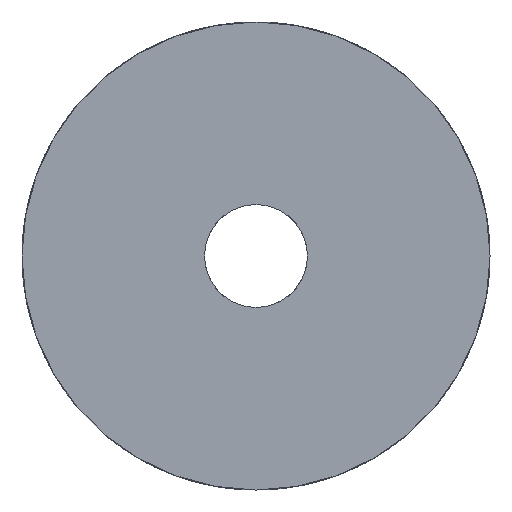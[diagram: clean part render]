
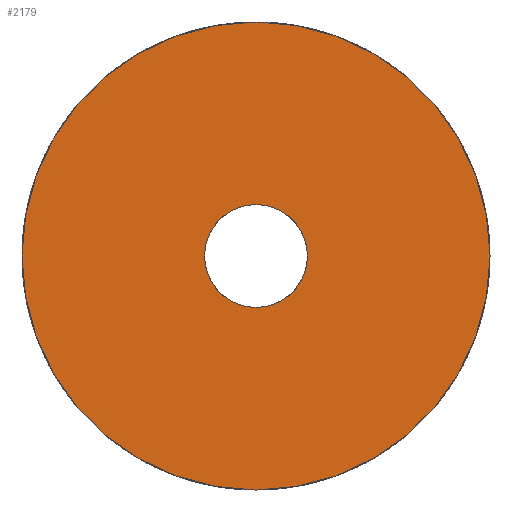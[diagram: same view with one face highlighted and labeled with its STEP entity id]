
A CAD part, front view. The second image highlights one B-rep face of the part: STEP entity #2179.
In plain terms, the highlighted planar face has unit normal (0, -1, 0).
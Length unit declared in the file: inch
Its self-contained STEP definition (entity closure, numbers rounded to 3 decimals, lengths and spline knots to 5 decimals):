
#25=PLANE('',#2441);
#343=FACE_BOUND('',#724,.T.);
#561=FACE_OUTER_BOUND('',#723,.T.);
#723=EDGE_LOOP('',(#1977));
#724=EDGE_LOOP('',(#1978));
#727=CIRCLE('',#2184,0.5);
#756=CIRCLE('',#2437,0.11);
#757=VERTEX_POINT('',#3035);
#978=VERTEX_POINT('',#5461);
#979=EDGE_CURVE('',#757,#757,#727,.T.);
#1312=EDGE_CURVE('',#978,#978,#756,.T.);
#1977=ORIENTED_EDGE('',*,*,#979,.F.);
#1978=ORIENTED_EDGE('',*,*,#1312,.T.);
#2179=ADVANCED_FACE('',(#561,#343),#25,.F.);
#2184=AXIS2_PLACEMENT_3D('',#3036,#2447,#2448);
#2437=AXIS2_PLACEMENT_3D('',#5462,#3021,#3022);
#2441=AXIS2_PLACEMENT_3D('',#5466,#3029,#3030);
#2447=DIRECTION('center_axis',(0.,1.,0.));
#2448=DIRECTION('ref_axis',(-1.,0.,0.));
#3021=DIRECTION('center_axis',(0.,1.,0.));
#3022=DIRECTION('ref_axis',(-1.,0.,0.));
#3029=DIRECTION('center_axis',(0.,1.,0.));
#3030=DIRECTION('ref_axis',(0.,0.,1.));
#3035=CARTESIAN_POINT('',(-0.5,0.,0.));
#3036=CARTESIAN_POINT('Origin',(0.,0.,0.));
#5461=CARTESIAN_POINT('',(0.11,0.,0.));
#5462=CARTESIAN_POINT('Origin',(0.,0.,0.));
#5466=CARTESIAN_POINT('Origin',(0.,0.,0.));
